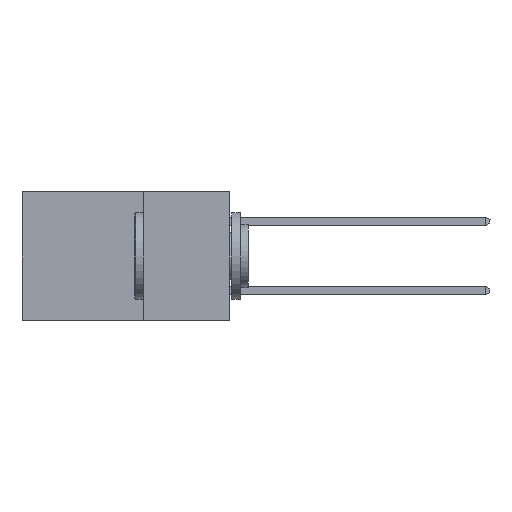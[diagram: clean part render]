
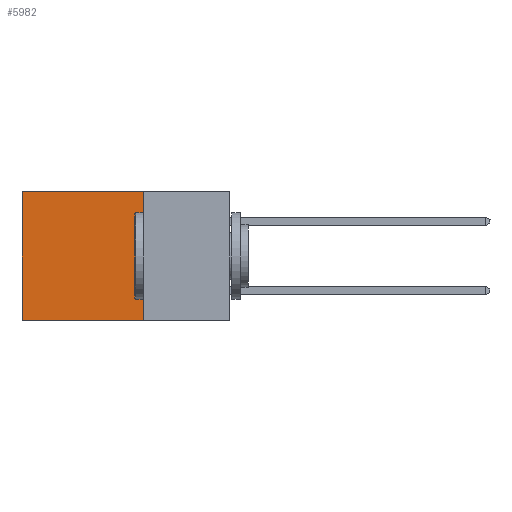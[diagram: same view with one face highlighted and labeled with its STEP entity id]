
A CAD part, left-side view. The second image highlights one B-rep face of the part: STEP entity #5982.
In plain terms, the highlighted planar face has unit normal (-1, 0, 0).
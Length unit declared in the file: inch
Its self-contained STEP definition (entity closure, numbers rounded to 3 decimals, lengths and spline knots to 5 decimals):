
#959 = DIRECTION ( 'NONE',  ( 0., 0., -1. ) ) ;
#1290 = ORIENTED_EDGE ( 'NONE', *, *, #16417, .F. ) ;
#1579 = VECTOR ( 'NONE', #6045, 39.37008 ) ;
#1858 = FACE_OUTER_BOUND ( 'NONE', #6336, .T. ) ;
#2064 = VERTEX_POINT ( 'NONE', #4531 ) ;
#2351 = CARTESIAN_POINT ( 'NONE',  ( 0.2615, 0.6, -0.37 ) ) ;
#3179 = CARTESIAN_POINT ( 'NONE',  ( 0.2615, 0.25, -0.37 ) ) ;
#4043 = AXIS2_PLACEMENT_3D ( 'NONE', #15571, #12326, #7889 ) ;
#4531 = CARTESIAN_POINT ( 'NONE',  ( 0.2615, 0.25, 0. ) ) ;
#5110 = LINE ( 'NONE', #12901, #11939 ) ;
#5982 = ADVANCED_FACE ( 'NONE', ( #1858 ), #9571, .F. ) ;
#6045 = DIRECTION ( 'NONE',  ( 0., 0., -1. ) ) ;
#6336 = EDGE_LOOP ( 'NONE', ( #15335, #1290, #18979, #12673 ) ) ;
#6784 = VERTEX_POINT ( 'NONE', #13631 ) ;
#6883 = LINE ( 'NONE', #14576, #7127 ) ;
#7127 = VECTOR ( 'NONE', #959, 39.37008 ) ;
#7889 = DIRECTION ( 'NONE',  ( 0., 0., -1. ) ) ;
#9105 = EDGE_CURVE ( 'NONE', #15886, #15950, #6883, .T. ) ;
#9571 = PLANE ( 'NONE',  #4043 ) ;
#10783 = LINE ( 'NONE', #3179, #1579 ) ;
#11551 = CARTESIAN_POINT ( 'NONE',  ( 0.2615, 0.6, 0. ) ) ;
#11719 = EDGE_CURVE ( 'NONE', #2064, #15886, #15665, .T. ) ;
#11939 = VECTOR ( 'NONE', #15851, 39.37008 ) ;
#12326 = DIRECTION ( 'NONE',  ( 1., 0., 0. ) ) ;
#12673 = ORIENTED_EDGE ( 'NONE', *, *, #11719, .T. ) ;
#12710 = DIRECTION ( 'NONE',  ( 0., 1., 0. ) ) ;
#12901 = CARTESIAN_POINT ( 'NONE',  ( 0.2615, 0.25, -0.37 ) ) ;
#13631 = CARTESIAN_POINT ( 'NONE',  ( 0.2615, 0.25, -0.37 ) ) ;
#14576 = CARTESIAN_POINT ( 'NONE',  ( 0.2615, 0.6, -0.37 ) ) ;
#15335 = ORIENTED_EDGE ( 'NONE', *, *, #9105, .T. ) ;
#15571 = CARTESIAN_POINT ( 'NONE',  ( 0.2615, 0.25, -0.37 ) ) ;
#15665 = LINE ( 'NONE', #17248, #15943 ) ;
#15851 = DIRECTION ( 'NONE',  ( 0., 1., 0. ) ) ;
#15886 = VERTEX_POINT ( 'NONE', #11551 ) ;
#15943 = VECTOR ( 'NONE', #12710, 39.37008 ) ;
#15950 = VERTEX_POINT ( 'NONE', #2351 ) ;
#16417 = EDGE_CURVE ( 'NONE', #6784, #15950, #5110, .T. ) ;
#17248 = CARTESIAN_POINT ( 'NONE',  ( 0.2615, 0.25, 0. ) ) ;
#17653 = EDGE_CURVE ( 'NONE', #2064, #6784, #10783, .T. ) ;
#18979 = ORIENTED_EDGE ( 'NONE', *, *, #17653, .F. ) ;
